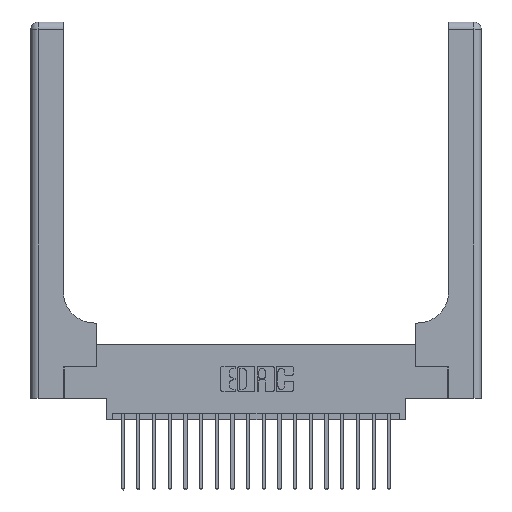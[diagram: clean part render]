
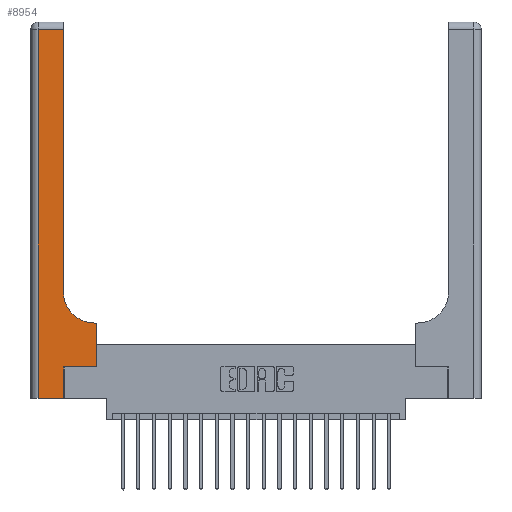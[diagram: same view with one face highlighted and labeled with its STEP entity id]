
A CAD part, top view. The second image highlights one B-rep face of the part: STEP entity #8954.
In plain terms, the highlighted planar face has unit normal (0, 0, 1).
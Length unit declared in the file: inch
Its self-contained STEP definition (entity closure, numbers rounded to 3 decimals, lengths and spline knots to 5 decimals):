
#241 = ORIENTED_EDGE ( 'NONE', *, *, #13206, .T. ) ;
#885 = CARTESIAN_POINT ( 'NONE',  ( 0.265, 0., 0.37 ) ) ;
#989 = ORIENTED_EDGE ( 'NONE', *, *, #16072, .T. ) ;
#1366 = VECTOR ( 'NONE', #1878, 39.37008 ) ;
#1567 = CARTESIAN_POINT ( 'NONE',  ( 0.26, 2.94, 0.37 ) ) ;
#1878 = DIRECTION ( 'NONE',  ( 0., -1., 0. ) ) ;
#2021 = LINE ( 'NONE', #11674, #9429 ) ;
#2135 = CARTESIAN_POINT ( 'NONE',  ( 0.528, 0.25, 0.37 ) ) ;
#2246 = DIRECTION ( 'NONE',  ( -1., 0., 0. ) ) ;
#2464 = EDGE_CURVE ( 'NONE', #12330, #3756, #8776, .T. ) ;
#2688 = DIRECTION ( 'NONE',  ( 0., 1., 0. ) ) ;
#2828 = EDGE_CURVE ( 'NONE', #11671, #10857, #11624, .T. ) ;
#2882 = CIRCLE ( 'NONE', #15719, 0.25 ) ;
#3756 = VERTEX_POINT ( 'NONE', #10010 ) ;
#4131 = VECTOR ( 'NONE', #10406, 39.37008 ) ;
#5621 = DIRECTION ( 'NONE',  ( 0., 1., 0. ) ) ;
#6546 = CARTESIAN_POINT ( 'NONE',  ( 0.265, 0., 0.37 ) ) ;
#6743 = AXIS2_PLACEMENT_3D ( 'NONE', #8394, #19272, #9938 ) ;
#7005 = DIRECTION ( 'NONE',  ( 0., 0., -1. ) ) ;
#7474 = CARTESIAN_POINT ( 'NONE',  ( 0.265, 0.25, 0.37 ) ) ;
#7488 = CARTESIAN_POINT ( 'NONE',  ( 0.26, 0.85, 0.37 ) ) ;
#7621 = EDGE_CURVE ( 'NONE', #3756, #11671, #20194, .T. ) ;
#7720 = ORIENTED_EDGE ( 'NONE', *, *, #13717, .T. ) ;
#8244 = LINE ( 'NONE', #19424, #16059 ) ;
#8249 = VERTEX_POINT ( 'NONE', #10865 ) ;
#8392 = ORIENTED_EDGE ( 'NONE', *, *, #19050, .T. ) ;
#8394 = CARTESIAN_POINT ( 'NONE',  ( 0., 3., 0.37 ) ) ;
#8776 = LINE ( 'NONE', #885, #12890 ) ;
#8813 = CARTESIAN_POINT ( 'NONE',  ( 0.26, 0.6, 0.37 ) ) ;
#8951 = VERTEX_POINT ( 'NONE', #14577 ) ;
#8954 = ADVANCED_FACE ( 'NONE', ( #19404 ), #17712, .F. ) ;
#9122 = ORIENTED_EDGE ( 'NONE', *, *, #7621, .T. ) ;
#9429 = VECTOR ( 'NONE', #2246, 39.37008 ) ;
#9938 = DIRECTION ( 'NONE',  ( -1., 0., 0. ) ) ;
#9939 = EDGE_CURVE ( 'NONE', #19230, #8951, #2021, .T. ) ;
#9959 = CARTESIAN_POINT ( 'NONE',  ( 0.528, 0.25, 0.37 ) ) ;
#10010 = CARTESIAN_POINT ( 'NONE',  ( 0.265, 0.25, 0.37 ) ) ;
#10406 = DIRECTION ( 'NONE',  ( -1., 0., 0. ) ) ;
#10630 = VECTOR ( 'NONE', #14687, 39.37008 ) ;
#10857 = VERTEX_POINT ( 'NONE', #18698 ) ;
#10865 = CARTESIAN_POINT ( 'NONE',  ( 0.06, 0., 0.37 ) ) ;
#11624 = LINE ( 'NONE', #2135, #10630 ) ;
#11671 = VERTEX_POINT ( 'NONE', #9959 ) ;
#11674 = CARTESIAN_POINT ( 'NONE',  ( 0., 2.94, 0.37 ) ) ;
#11912 = VECTOR ( 'NONE', #15339, 39.37008 ) ;
#12330 = VERTEX_POINT ( 'NONE', #6546 ) ;
#12890 = VECTOR ( 'NONE', #5621, 39.37008 ) ;
#13206 = EDGE_CURVE ( 'NONE', #18669, #16301, #2882, .T. ) ;
#13215 = ORIENTED_EDGE ( 'NONE', *, *, #2828, .T. ) ;
#13325 = EDGE_CURVE ( 'NONE', #10857, #18669, #16616, .T. ) ;
#13329 = LINE ( 'NONE', #19914, #20153 ) ;
#13717 = EDGE_CURVE ( 'NONE', #8951, #8249, #13901, .T. ) ;
#13901 = LINE ( 'NONE', #14423, #1366 ) ;
#14423 = CARTESIAN_POINT ( 'NONE',  ( 0.06, 3., 0.37 ) ) ;
#14577 = CARTESIAN_POINT ( 'NONE',  ( 0.06, 2.94, 0.37 ) ) ;
#14687 = DIRECTION ( 'NONE',  ( 0., 1., 0. ) ) ;
#14699 = ORIENTED_EDGE ( 'NONE', *, *, #13325, .T. ) ;
#15339 = DIRECTION ( 'NONE',  ( 1., 0., 0. ) ) ;
#15719 = AXIS2_PLACEMENT_3D ( 'NONE', #16376, #7005, #17917 ) ;
#16059 = VECTOR ( 'NONE', #17868, 39.37008 ) ;
#16072 = EDGE_CURVE ( 'NONE', #8249, #12330, #8244, .T. ) ;
#16080 = CARTESIAN_POINT ( 'NONE',  ( 0.51, 0.6, 0.37 ) ) ;
#16301 = VERTEX_POINT ( 'NONE', #7488 ) ;
#16376 = CARTESIAN_POINT ( 'NONE',  ( 0.51, 0.85, 0.37 ) ) ;
#16616 = LINE ( 'NONE', #8813, #4131 ) ;
#16696 = ORIENTED_EDGE ( 'NONE', *, *, #9939, .T. ) ;
#17024 = EDGE_LOOP ( 'NONE', ( #8392, #16696, #7720, #989, #18486, #9122, #13215, #14699, #241 ) ) ;
#17712 = PLANE ( 'NONE',  #6743 ) ;
#17868 = DIRECTION ( 'NONE',  ( 1., 0., 0. ) ) ;
#17917 = DIRECTION ( 'NONE',  ( 1., 0., 0. ) ) ;
#18486 = ORIENTED_EDGE ( 'NONE', *, *, #2464, .T. ) ;
#18669 = VERTEX_POINT ( 'NONE', #16080 ) ;
#18698 = CARTESIAN_POINT ( 'NONE',  ( 0.528, 0.6, 0.37 ) ) ;
#19050 = EDGE_CURVE ( 'NONE', #16301, #19230, #13329, .T. ) ;
#19230 = VERTEX_POINT ( 'NONE', #1567 ) ;
#19272 = DIRECTION ( 'NONE',  ( 0., 0., -1. ) ) ;
#19404 = FACE_OUTER_BOUND ( 'NONE', #17024, .T. ) ;
#19424 = CARTESIAN_POINT ( 'NONE',  ( 0., 0., 0.37 ) ) ;
#19914 = CARTESIAN_POINT ( 'NONE',  ( 0.26, 3., 0.37 ) ) ;
#20153 = VECTOR ( 'NONE', #2688, 39.37008 ) ;
#20194 = LINE ( 'NONE', #7474, #11912 ) ;
